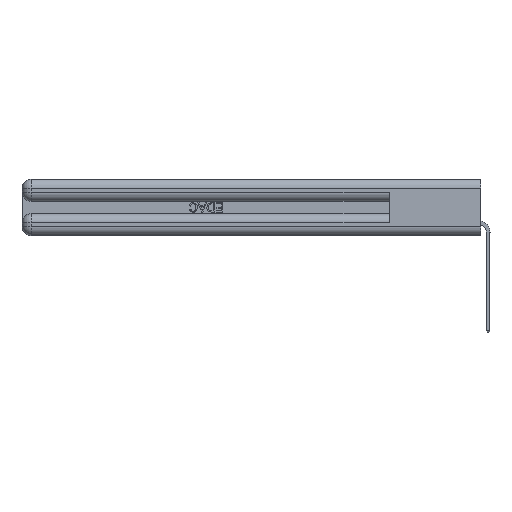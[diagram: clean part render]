
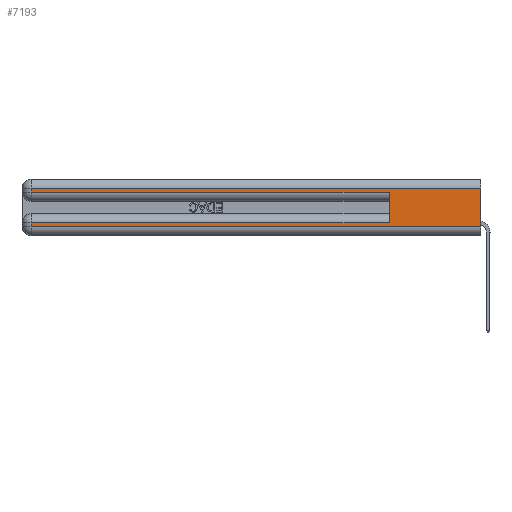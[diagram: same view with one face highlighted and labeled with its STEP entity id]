
A CAD part, left-side view. The second image highlights one B-rep face of the part: STEP entity #7193.
In plain terms, the highlighted planar face has unit normal (-1, 0, 0).
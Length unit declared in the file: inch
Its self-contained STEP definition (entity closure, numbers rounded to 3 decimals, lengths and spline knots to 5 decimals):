
#718 = VECTOR ( 'NONE', #32249, 39.37008 ) ;
#742 = EDGE_CURVE ( 'NONE', #36987, #12960, #16724, .T. ) ;
#1557 = ORIENTED_EDGE ( 'NONE', *, *, #16795, .T. ) ;
#2071 = EDGE_CURVE ( 'NONE', #40218, #29857, #37584, .T. ) ;
#2340 = DIRECTION ( 'NONE',  ( 1., 0., 0. ) ) ;
#2708 = EDGE_CURVE ( 'NONE', #33648, #3768, #38038, .T. ) ;
#3307 = DIRECTION ( 'NONE',  ( 0., 0., -1. ) ) ;
#3323 = CARTESIAN_POINT ( 'NONE',  ( 0., 2.94, 0.06 ) ) ;
#3768 = VERTEX_POINT ( 'NONE', #24403 ) ;
#3930 = CARTESIAN_POINT ( 'NONE',  ( 0., 0.6, 0.085 ) ) ;
#4534 = DIRECTION ( 'NONE',  ( 0., 1., 0. ) ) ;
#5098 = CARTESIAN_POINT ( 'NONE',  ( 0., 0., 0.37 ) ) ;
#5213 = VECTOR ( 'NONE', #6702, 39.37008 ) ;
#6338 = ORIENTED_EDGE ( 'NONE', *, *, #2071, .F. ) ;
#6702 = DIRECTION ( 'NONE',  ( 0., 0., 1. ) ) ;
#7193 = ADVANCED_FACE ( 'NONE', ( #14055 ), #36804, .F. ) ;
#7286 = CARTESIAN_POINT ( 'NONE',  ( 0., 0., 0.085 ) ) ;
#7597 = CARTESIAN_POINT ( 'NONE',  ( 0., 0., 0.06 ) ) ;
#7756 = VECTOR ( 'NONE', #3307, 39.37008 ) ;
#7949 = CARTESIAN_POINT ( 'NONE',  ( 0., 2.94, 0.37 ) ) ;
#8112 = DIRECTION ( 'NONE',  ( 0., 0., -1. ) ) ;
#8294 = CARTESIAN_POINT ( 'NONE',  ( 0., 0., 0.06 ) ) ;
#8396 = CARTESIAN_POINT ( 'NONE',  ( 0., 0., 0.37 ) ) ;
#8801 = ORIENTED_EDGE ( 'NONE', *, *, #37041, .T. ) ;
#8833 = CARTESIAN_POINT ( 'NONE',  ( 0., 0., 0.31 ) ) ;
#9154 = VECTOR ( 'NONE', #16509, 39.37008 ) ;
#9338 = ORIENTED_EDGE ( 'NONE', *, *, #15942, .F. ) ;
#11703 = VECTOR ( 'NONE', #4534, 39.37008 ) ;
#12305 = VERTEX_POINT ( 'NONE', #8833 ) ;
#12622 = LINE ( 'NONE', #15876, #9154 ) ;
#12721 = LINE ( 'NONE', #35024, #7756 ) ;
#12960 = VERTEX_POINT ( 'NONE', #8294 ) ;
#13245 = CARTESIAN_POINT ( 'NONE',  ( 0., 0.6, 0.145 ) ) ;
#14055 = FACE_OUTER_BOUND ( 'NONE', #24832, .T. ) ;
#14770 = ORIENTED_EDGE ( 'NONE', *, *, #29905, .T. ) ;
#15876 = CARTESIAN_POINT ( 'NONE',  ( 0., 0., 0.31 ) ) ;
#15942 = EDGE_CURVE ( 'NONE', #12305, #12960, #35284, .T. ) ;
#16385 = CARTESIAN_POINT ( 'NONE',  ( 0., 0., 0.285 ) ) ;
#16509 = DIRECTION ( 'NONE',  ( 0., 1., 0. ) ) ;
#16724 = LINE ( 'NONE', #7597, #23181 ) ;
#16795 = EDGE_CURVE ( 'NONE', #12305, #33648, #12622, .T. ) ;
#17217 = DIRECTION ( 'NONE',  ( 0., -1., 0. ) ) ;
#18373 = VERTEX_POINT ( 'NONE', #40065 ) ;
#19599 = LINE ( 'NONE', #7286, #11703 ) ;
#20430 = DIRECTION ( 'NONE',  ( 0., 0., -1. ) ) ;
#21364 = AXIS2_PLACEMENT_3D ( 'NONE', #5098, #2340, #27779 ) ;
#21868 = EDGE_CURVE ( 'NONE', #18373, #36987, #12721, .T. ) ;
#23181 = VECTOR ( 'NONE', #17217, 39.37008 ) ;
#24296 = ORIENTED_EDGE ( 'NONE', *, *, #21868, .T. ) ;
#24403 = CARTESIAN_POINT ( 'NONE',  ( 0., 2.94, 0.285 ) ) ;
#24832 = EDGE_LOOP ( 'NONE', ( #9338, #1557, #36493, #8801, #6338, #14770, #24296, #31541 ) ) ;
#25514 = CARTESIAN_POINT ( 'NONE',  ( 0., 0.6, 0.285 ) ) ;
#27405 = CARTESIAN_POINT ( 'NONE',  ( 0., 2.94, 0.31 ) ) ;
#27563 = VECTOR ( 'NONE', #20430, 39.37008 ) ;
#27779 = DIRECTION ( 'NONE',  ( 0., 0., -1. ) ) ;
#29857 = VERTEX_POINT ( 'NONE', #25514 ) ;
#29905 = EDGE_CURVE ( 'NONE', #40218, #18373, #19599, .T. ) ;
#31214 = LINE ( 'NONE', #16385, #718 ) ;
#31541 = ORIENTED_EDGE ( 'NONE', *, *, #742, .T. ) ;
#32249 = DIRECTION ( 'NONE',  ( 0., -1., 0. ) ) ;
#33648 = VERTEX_POINT ( 'NONE', #27405 ) ;
#35024 = CARTESIAN_POINT ( 'NONE',  ( 0., 2.94, 0.37 ) ) ;
#35284 = LINE ( 'NONE', #8396, #40378 ) ;
#36493 = ORIENTED_EDGE ( 'NONE', *, *, #2708, .T. ) ;
#36804 = PLANE ( 'NONE',  #21364 ) ;
#36987 = VERTEX_POINT ( 'NONE', #3323 ) ;
#37041 = EDGE_CURVE ( 'NONE', #3768, #29857, #31214, .T. ) ;
#37584 = LINE ( 'NONE', #13245, #5213 ) ;
#38038 = LINE ( 'NONE', #7949, #27563 ) ;
#40065 = CARTESIAN_POINT ( 'NONE',  ( 0., 2.94, 0.085 ) ) ;
#40218 = VERTEX_POINT ( 'NONE', #3930 ) ;
#40378 = VECTOR ( 'NONE', #8112, 39.37008 ) ;
